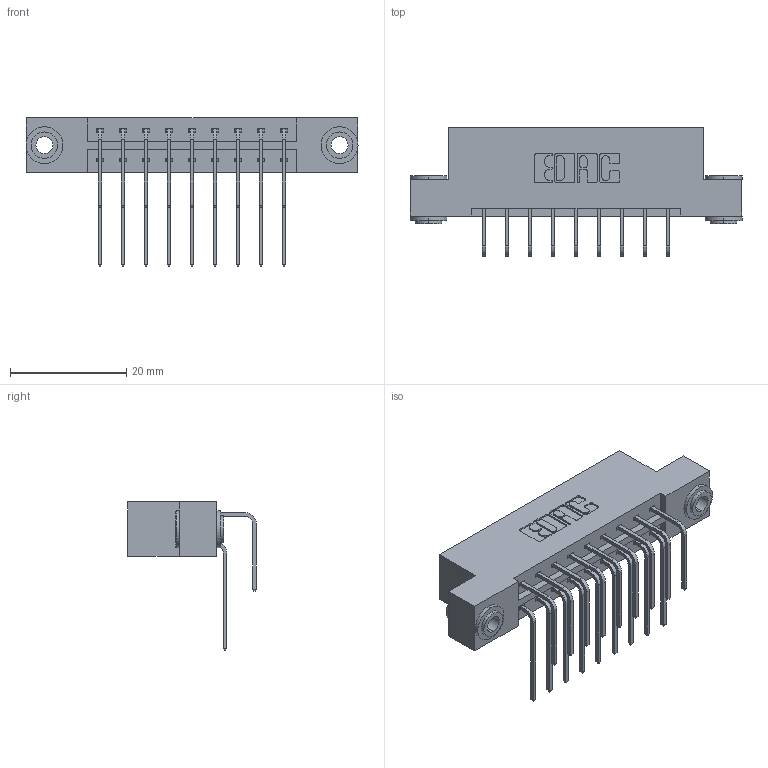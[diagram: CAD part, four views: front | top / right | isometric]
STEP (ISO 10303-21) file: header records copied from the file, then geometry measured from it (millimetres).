
FILE_DESCRIPTION (( 'STEP AP203' ), '1' );
FILE_NAME ('333-018-558-203.STEP', '2019-08-09T14:10:25', ( '' ), ( '' ), 'SwSTEP 2.0', 'SolidWorks 2016', '' );
FILE_SCHEMA (( 'CONFIG_CONTROL_DESIGN' ));
Length unit declared in the file: inch
Products named in the file (5): 333-018-558-203; 333 Part_Flush - .156 Dia - TH; 345-292-001_558 Tail - 2; 345-250-002_345-250-002-102; 345-292-001_558 559 Tail - 1
Assembly tree (21 placements, depth 2):
  333-018-558-203
    333 Part_Flush - .156 Dia - TH
    345-292-001_558 559 Tail - 1  x9
    345-292-001_558 Tail - 2  x9
    345-250-002_345-250-002-102  x2
Bounding box: 57.2 x 22.17 x 25.53 mm (x, y, z)
Volume: 5654.5 mm3; surface area: 7068.5 mm2
Topology: 21 solids, 21 shells, 1124 faces, 3285 edges, 2162 vertices
Faces by surface type: plane 764, cylinder 352, cone 8
Entity records: 12492 total; most frequent: CARTESIAN_POINT 2136, ORIENTED_EDGE 2014, DIRECTION 1897, EDGE_CURVE 1007, VECTOR 815, LINE 815, VERTEX_POINT 666, AXIS2_PLACEMENT_3D 541
